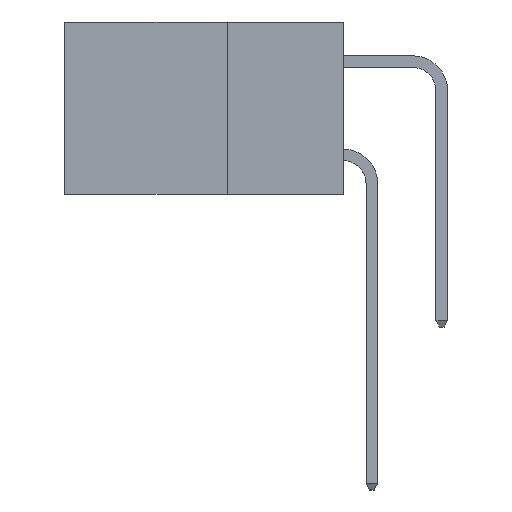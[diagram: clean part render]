
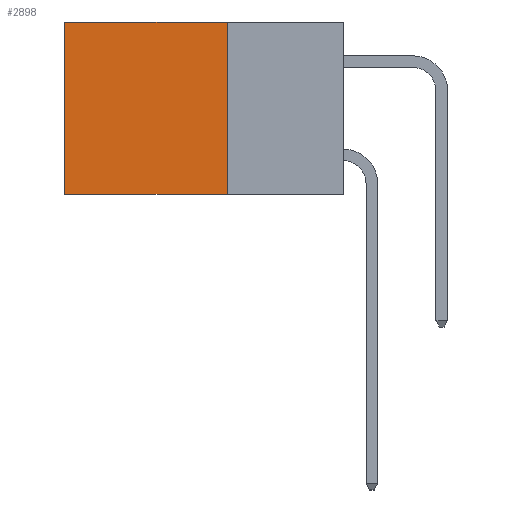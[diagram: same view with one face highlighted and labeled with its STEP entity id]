
A CAD part, left-side view. The second image highlights one B-rep face of the part: STEP entity #2898.
In plain terms, the highlighted planar face has unit normal (-1, 0, 0).
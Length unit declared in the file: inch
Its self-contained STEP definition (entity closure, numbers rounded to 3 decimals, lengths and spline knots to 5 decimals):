
#702 = EDGE_LOOP ( 'NONE', ( #11404, #7236, #13268, #2675 ) ) ;
#771 = VECTOR ( 'NONE', #8023, 39.37008 ) ;
#904 = DIRECTION ( 'NONE',  ( 0., 0., -1. ) ) ;
#925 = DIRECTION ( 'NONE',  ( 1., 0., 0. ) ) ;
#947 = PLANE ( 'NONE',  #4392 ) ;
#1048 = CARTESIAN_POINT ( 'NONE',  ( 0.2615, 0.25, -0.37 ) ) ;
#1608 = LINE ( 'NONE', #11894, #12294 ) ;
#1857 = EDGE_CURVE ( 'NONE', #2798, #6688, #14287, .T. ) ;
#2072 = CARTESIAN_POINT ( 'NONE',  ( 0.2615, 0.6, -0.37 ) ) ;
#2159 = DIRECTION ( 'NONE',  ( 0., 1., 0. ) ) ;
#2675 = ORIENTED_EDGE ( 'NONE', *, *, #3861, .T. ) ;
#2717 = CARTESIAN_POINT ( 'NONE',  ( 0.2615, 0.6, 0. ) ) ;
#2798 = VERTEX_POINT ( 'NONE', #2717 ) ;
#2898 = ADVANCED_FACE ( 'NONE', ( #16723 ), #947, .F. ) ;
#3814 = VERTEX_POINT ( 'NONE', #9005 ) ;
#3861 = EDGE_CURVE ( 'NONE', #3814, #2798, #6126, .T. ) ;
#4392 = AXIS2_PLACEMENT_3D ( 'NONE', #1048, #925, #904 ) ;
#6126 = LINE ( 'NONE', #8382, #13361 ) ;
#6658 = CARTESIAN_POINT ( 'NONE',  ( 0.2615, 0.25, -0.37 ) ) ;
#6688 = VERTEX_POINT ( 'NONE', #2072 ) ;
#7236 = ORIENTED_EDGE ( 'NONE', *, *, #17341, .F. ) ;
#8023 = DIRECTION ( 'NONE',  ( 0., 0., -1. ) ) ;
#8230 = DIRECTION ( 'NONE',  ( 0., 1., 0. ) ) ;
#8382 = CARTESIAN_POINT ( 'NONE',  ( 0.2615, 0.25, 0. ) ) ;
#9005 = CARTESIAN_POINT ( 'NONE',  ( 0.2615, 0.25, 0. ) ) ;
#10007 = CARTESIAN_POINT ( 'NONE',  ( 0.2615, 0.25, -0.37 ) ) ;
#11404 = ORIENTED_EDGE ( 'NONE', *, *, #1857, .T. ) ;
#11799 = EDGE_CURVE ( 'NONE', #3814, #16462, #11928, .T. ) ;
#11894 = CARTESIAN_POINT ( 'NONE',  ( 0.2615, 0.25, -0.37 ) ) ;
#11928 = LINE ( 'NONE', #6658, #771 ) ;
#12294 = VECTOR ( 'NONE', #2159, 39.37008 ) ;
#13268 = ORIENTED_EDGE ( 'NONE', *, *, #11799, .F. ) ;
#13361 = VECTOR ( 'NONE', #8230, 39.37008 ) ;
#14287 = LINE ( 'NONE', #15829, #17184 ) ;
#15829 = CARTESIAN_POINT ( 'NONE',  ( 0.2615, 0.6, -0.37 ) ) ;
#16462 = VERTEX_POINT ( 'NONE', #10007 ) ;
#16723 = FACE_OUTER_BOUND ( 'NONE', #702, .T. ) ;
#16839 = DIRECTION ( 'NONE',  ( 0., 0., -1. ) ) ;
#17184 = VECTOR ( 'NONE', #16839, 39.37008 ) ;
#17341 = EDGE_CURVE ( 'NONE', #16462, #6688, #1608, .T. ) ;
